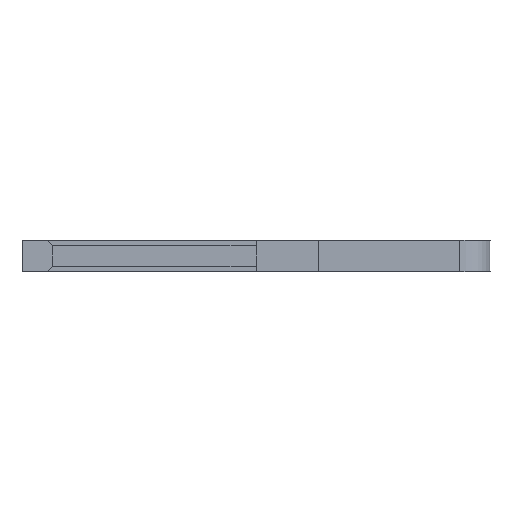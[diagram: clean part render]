
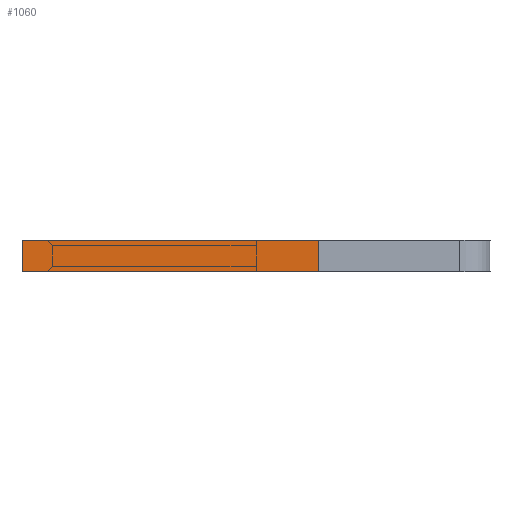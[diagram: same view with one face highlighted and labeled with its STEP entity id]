
A CAD part, left-side view. The second image highlights one B-rep face of the part: STEP entity #1060.
In plain terms, the highlighted face is planar.
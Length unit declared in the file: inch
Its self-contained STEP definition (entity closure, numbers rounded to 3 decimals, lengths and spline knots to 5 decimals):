
#106 = CARTESIAN_POINT ( 'NONE',  ( -0.01, -0.04, -0.04 ) ) ;
#509 = VERTEX_POINT ( 'NONE', #2823 ) ;
#706 = CARTESIAN_POINT ( 'NONE',  ( 0.01, 0.15, -0.04 ) ) ;
#795 = VECTOR ( 'NONE', #3071, 39.37008 ) ;
#873 = DIRECTION ( 'NONE',  ( 1., 0., 0. ) ) ;
#1060 = ADVANCED_FACE ( 'NONE', ( #3333 ), #1576, .F. ) ;
#1193 = CARTESIAN_POINT ( 'NONE',  ( 0.01, 0.15, -0.04 ) ) ;
#1413 = EDGE_LOOP ( 'NONE', ( #3870, #1546, #1616, #2011 ) ) ;
#1519 = EDGE_CURVE ( 'NONE', #4131, #2653, #3230, .T. ) ;
#1546 = ORIENTED_EDGE ( 'NONE', *, *, #3584, .F. ) ;
#1576 = PLANE ( 'NONE',  #2669 ) ;
#1616 = ORIENTED_EDGE ( 'NONE', *, *, #1519, .F. ) ;
#1622 = LINE ( 'NONE', #3712, #3208 ) ;
#1835 = CARTESIAN_POINT ( 'NONE',  ( 0.01, -0.04, -0.04 ) ) ;
#1866 = DIRECTION ( 'NONE',  ( 0., 0., 1. ) ) ;
#1899 = LINE ( 'NONE', #1835, #2056 ) ;
#1975 = CARTESIAN_POINT ( 'NONE',  ( 0.01, 0.15, -0.04 ) ) ;
#2011 = ORIENTED_EDGE ( 'NONE', *, *, #3943, .T. ) ;
#2056 = VECTOR ( 'NONE', #4207, 39.37008 ) ;
#2269 = EDGE_CURVE ( 'NONE', #2921, #509, #1622, .T. ) ;
#2271 = LINE ( 'NONE', #706, #795 ) ;
#2653 = VERTEX_POINT ( 'NONE', #3740 ) ;
#2669 = AXIS2_PLACEMENT_3D ( 'NONE', #1193, #1866, #873 ) ;
#2701 = DIRECTION ( 'NONE',  ( 0., 1., 0. ) ) ;
#2823 = CARTESIAN_POINT ( 'NONE',  ( -0.01, 0.15, -0.04 ) ) ;
#2852 = CARTESIAN_POINT ( 'NONE',  ( 0.01, -0.04, -0.04 ) ) ;
#2921 = VERTEX_POINT ( 'NONE', #106 ) ;
#3071 = DIRECTION ( 'NONE',  ( -1., 0., 0. ) ) ;
#3208 = VECTOR ( 'NONE', #2701, 39.37008 ) ;
#3230 = LINE ( 'NONE', #1975, #4022 ) ;
#3333 = FACE_OUTER_BOUND ( 'NONE', #1413, .T. ) ;
#3584 = EDGE_CURVE ( 'NONE', #2653, #509, #2271, .T. ) ;
#3628 = DIRECTION ( 'NONE',  ( 0., 1., 0. ) ) ;
#3712 = CARTESIAN_POINT ( 'NONE',  ( -0.01, 0.15, -0.04 ) ) ;
#3740 = CARTESIAN_POINT ( 'NONE',  ( 0.01, 0.15, -0.04 ) ) ;
#3870 = ORIENTED_EDGE ( 'NONE', *, *, #2269, .T. ) ;
#3943 = EDGE_CURVE ( 'NONE', #4131, #2921, #1899, .T. ) ;
#4022 = VECTOR ( 'NONE', #3628, 39.37008 ) ;
#4131 = VERTEX_POINT ( 'NONE', #2852 ) ;
#4207 = DIRECTION ( 'NONE',  ( -1., 0., 0. ) ) ;
